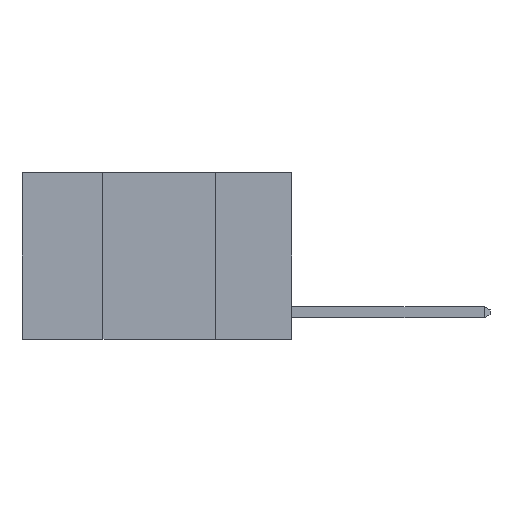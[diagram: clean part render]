
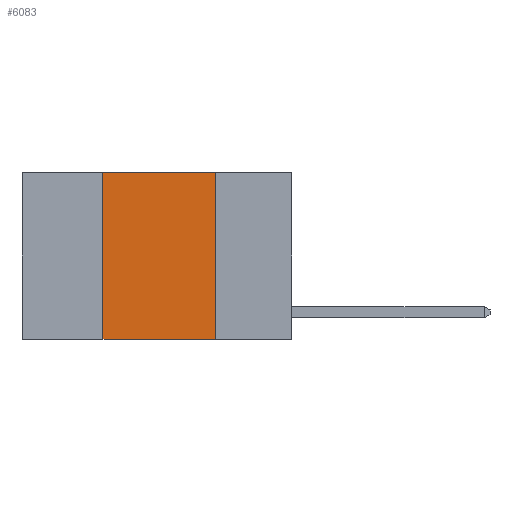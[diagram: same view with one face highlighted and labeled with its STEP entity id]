
A CAD part, left-side view. The second image highlights one B-rep face of the part: STEP entity #6083.
In plain terms, the highlighted planar face has unit normal (-1, 0, 0).
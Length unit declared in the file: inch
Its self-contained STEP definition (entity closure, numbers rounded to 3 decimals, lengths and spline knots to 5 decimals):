
#68 = LINE ( 'NONE', #3931, #2395 ) ;
#122 = LINE ( 'NONE', #6243, #4437 ) ;
#206 = CARTESIAN_POINT ( 'NONE',  ( 0., 0.42, 0. ) ) ;
#781 = ORIENTED_EDGE ( 'NONE', *, *, #6402, .F. ) ;
#1562 = CARTESIAN_POINT ( 'NONE',  ( 0., 0.42, 0. ) ) ;
#1782 = VERTEX_POINT ( 'NONE', #5494 ) ;
#1906 = ORIENTED_EDGE ( 'NONE', *, *, #7016, .F. ) ;
#1974 = LINE ( 'NONE', #3901, #6168 ) ;
#2301 = VERTEX_POINT ( 'NONE', #2842 ) ;
#2395 = VECTOR ( 'NONE', #7999, 39.37008 ) ;
#2528 = ORIENTED_EDGE ( 'NONE', *, *, #9574, .F. ) ;
#2842 = CARTESIAN_POINT ( 'NONE',  ( 0., 0.42, -0.37 ) ) ;
#2898 = VERTEX_POINT ( 'NONE', #5254 ) ;
#2992 = ORIENTED_EDGE ( 'NONE', *, *, #3044, .T. ) ;
#3044 = EDGE_CURVE ( 'NONE', #2301, #1782, #68, .T. ) ;
#3086 = EDGE_LOOP ( 'NONE', ( #781, #2528, #1906, #2992 ) ) ;
#3250 = DIRECTION ( 'NONE',  ( 1., 0., 0. ) ) ;
#3737 = AXIS2_PLACEMENT_3D ( 'NONE', #6568, #3250, #8951 ) ;
#3901 = CARTESIAN_POINT ( 'NONE',  ( 0., 0.6, 0. ) ) ;
#3913 = FACE_OUTER_BOUND ( 'NONE', #3086, .T. ) ;
#3931 = CARTESIAN_POINT ( 'NONE',  ( 0., 0.6, -0.37 ) ) ;
#4437 = VECTOR ( 'NONE', #10182, 39.37008 ) ;
#4545 = VERTEX_POINT ( 'NONE', #1562 ) ;
#5254 = CARTESIAN_POINT ( 'NONE',  ( 0., 0.17, 0. ) ) ;
#5494 = CARTESIAN_POINT ( 'NONE',  ( 0., 0.17, -0.37 ) ) ;
#6083 = ADVANCED_FACE ( 'NONE', ( #3913 ), #7292, .F. ) ;
#6168 = VECTOR ( 'NONE', #8757, 39.37008 ) ;
#6243 = CARTESIAN_POINT ( 'NONE',  ( 0., 0.17, 0. ) ) ;
#6402 = EDGE_CURVE ( 'NONE', #2898, #1782, #122, .T. ) ;
#6568 = CARTESIAN_POINT ( 'NONE',  ( 0., 0.6, 0. ) ) ;
#6990 = VECTOR ( 'NONE', #7002, 39.37008 ) ;
#7002 = DIRECTION ( 'NONE',  ( 0., 0., 1. ) ) ;
#7016 = EDGE_CURVE ( 'NONE', #2301, #4545, #9085, .T. ) ;
#7292 = PLANE ( 'NONE',  #3737 ) ;
#7999 = DIRECTION ( 'NONE',  ( 0., -1., 0. ) ) ;
#8757 = DIRECTION ( 'NONE',  ( 0., -1., 0. ) ) ;
#8951 = DIRECTION ( 'NONE',  ( 0., 0., -1. ) ) ;
#9085 = LINE ( 'NONE', #206, #6990 ) ;
#9574 = EDGE_CURVE ( 'NONE', #4545, #2898, #1974, .T. ) ;
#10182 = DIRECTION ( 'NONE',  ( 0., 0., -1. ) ) ;
